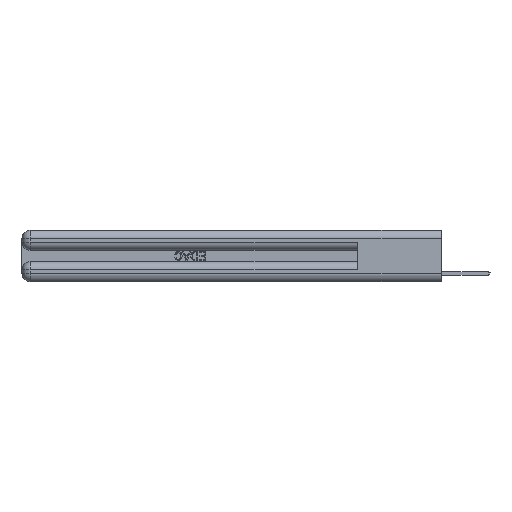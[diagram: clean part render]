
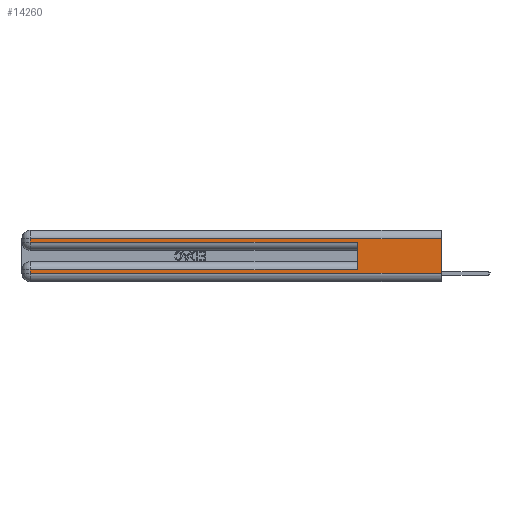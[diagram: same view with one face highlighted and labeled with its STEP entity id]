
A CAD part, left-side view. The second image highlights one B-rep face of the part: STEP entity #14260.
In plain terms, the highlighted planar face has unit normal (-1, 0, 0).
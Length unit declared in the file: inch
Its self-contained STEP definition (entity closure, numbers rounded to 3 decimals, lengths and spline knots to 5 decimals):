
#330 = CARTESIAN_POINT ( 'NONE',  ( 0., 0., 0.285 ) ) ;
#451 = LINE ( 'NONE', #746, #28197 ) ;
#746 = CARTESIAN_POINT ( 'NONE',  ( 0., 0.6, 0.145 ) ) ;
#761 = DIRECTION ( 'NONE',  ( 0., 1., 0. ) ) ;
#969 = VECTOR ( 'NONE', #25987, 39.37008 ) ;
#1002 = VERTEX_POINT ( 'NONE', #11687 ) ;
#1419 = LINE ( 'NONE', #12289, #25534 ) ;
#2130 = DIRECTION ( 'NONE',  ( 0., 0., -1. ) ) ;
#2794 = VERTEX_POINT ( 'NONE', #22962 ) ;
#2935 = LINE ( 'NONE', #11737, #20158 ) ;
#4661 = EDGE_CURVE ( 'NONE', #17708, #2794, #22642, .T. ) ;
#5091 = ORIENTED_EDGE ( 'NONE', *, *, #17138, .F. ) ;
#5491 = ORIENTED_EDGE ( 'NONE', *, *, #16500, .T. ) ;
#5612 = CARTESIAN_POINT ( 'NONE',  ( 0., 2.94, 0.37 ) ) ;
#5658 = CARTESIAN_POINT ( 'NONE',  ( 0., 0., 0.06 ) ) ;
#5917 = EDGE_CURVE ( 'NONE', #13812, #17708, #11836, .T. ) ;
#6360 = VECTOR ( 'NONE', #23069, 39.37008 ) ;
#7312 = ORIENTED_EDGE ( 'NONE', *, *, #24206, .T. ) ;
#7314 = AXIS2_PLACEMENT_3D ( 'NONE', #14499, #27528, #18728 ) ;
#7470 = VECTOR ( 'NONE', #761, 39.37008 ) ;
#8201 = CARTESIAN_POINT ( 'NONE',  ( 0., 0., 0.085 ) ) ;
#8239 = ORIENTED_EDGE ( 'NONE', *, *, #5917, .T. ) ;
#8325 = CARTESIAN_POINT ( 'NONE',  ( 0., 2.94, 0.285 ) ) ;
#10280 = CARTESIAN_POINT ( 'NONE',  ( 0., 0.6, 0.085 ) ) ;
#10772 = VECTOR ( 'NONE', #25434, 39.37008 ) ;
#11687 = CARTESIAN_POINT ( 'NONE',  ( 0., 2.94, 0.06 ) ) ;
#11737 = CARTESIAN_POINT ( 'NONE',  ( 0., 2.94, 0.37 ) ) ;
#11836 = LINE ( 'NONE', #5612, #10772 ) ;
#12018 = FACE_OUTER_BOUND ( 'NONE', #28008, .T. ) ;
#12289 = CARTESIAN_POINT ( 'NONE',  ( 0., 0., 0.37 ) ) ;
#12686 = EDGE_CURVE ( 'NONE', #17249, #1002, #2935, .T. ) ;
#13812 = VERTEX_POINT ( 'NONE', #17478 ) ;
#14260 = ADVANCED_FACE ( 'NONE', ( #12018 ), #23301, .F. ) ;
#14492 = DIRECTION ( 'NONE',  ( 0., -1., 0. ) ) ;
#14499 = CARTESIAN_POINT ( 'NONE',  ( 0., 0., 0.37 ) ) ;
#14530 = CARTESIAN_POINT ( 'NONE',  ( 0., 0., 0.06 ) ) ;
#15000 = LINE ( 'NONE', #8201, #969 ) ;
#16500 = EDGE_CURVE ( 'NONE', #24735, #17249, #15000, .T. ) ;
#16930 = CARTESIAN_POINT ( 'NONE',  ( 0., 0., 0.31 ) ) ;
#17124 = CARTESIAN_POINT ( 'NONE',  ( 0., 0., 0.31 ) ) ;
#17138 = EDGE_CURVE ( 'NONE', #26642, #23836, #1419, .T. ) ;
#17249 = VERTEX_POINT ( 'NONE', #27020 ) ;
#17478 = CARTESIAN_POINT ( 'NONE',  ( 0., 2.94, 0.31 ) ) ;
#17708 = VERTEX_POINT ( 'NONE', #8325 ) ;
#18728 = DIRECTION ( 'NONE',  ( 0., 0., -1. ) ) ;
#19186 = ORIENTED_EDGE ( 'NONE', *, *, #4661, .T. ) ;
#19221 = ORIENTED_EDGE ( 'NONE', *, *, #27101, .F. ) ;
#20158 = VECTOR ( 'NONE', #26962, 39.37008 ) ;
#20686 = LINE ( 'NONE', #17124, #7470 ) ;
#20938 = VECTOR ( 'NONE', #14492, 39.37008 ) ;
#21988 = EDGE_CURVE ( 'NONE', #26642, #13812, #20686, .T. ) ;
#22612 = DIRECTION ( 'NONE',  ( 0., 0., 1. ) ) ;
#22642 = LINE ( 'NONE', #330, #6360 ) ;
#22962 = CARTESIAN_POINT ( 'NONE',  ( 0., 0.6, 0.285 ) ) ;
#23069 = DIRECTION ( 'NONE',  ( 0., -1., 0. ) ) ;
#23301 = PLANE ( 'NONE',  #7314 ) ;
#23672 = ORIENTED_EDGE ( 'NONE', *, *, #12686, .T. ) ;
#23836 = VERTEX_POINT ( 'NONE', #14530 ) ;
#24203 = ORIENTED_EDGE ( 'NONE', *, *, #21988, .T. ) ;
#24206 = EDGE_CURVE ( 'NONE', #1002, #23836, #25754, .T. ) ;
#24735 = VERTEX_POINT ( 'NONE', #10280 ) ;
#25434 = DIRECTION ( 'NONE',  ( 0., 0., -1. ) ) ;
#25534 = VECTOR ( 'NONE', #2130, 39.37008 ) ;
#25754 = LINE ( 'NONE', #5658, #20938 ) ;
#25987 = DIRECTION ( 'NONE',  ( 0., 1., 0. ) ) ;
#26642 = VERTEX_POINT ( 'NONE', #16930 ) ;
#26962 = DIRECTION ( 'NONE',  ( 0., 0., -1. ) ) ;
#27020 = CARTESIAN_POINT ( 'NONE',  ( 0., 2.94, 0.085 ) ) ;
#27101 = EDGE_CURVE ( 'NONE', #24735, #2794, #451, .T. ) ;
#27528 = DIRECTION ( 'NONE',  ( 1., 0., 0. ) ) ;
#28008 = EDGE_LOOP ( 'NONE', ( #5091, #24203, #8239, #19186, #19221, #5491, #23672, #7312 ) ) ;
#28197 = VECTOR ( 'NONE', #22612, 39.37008 ) ;
